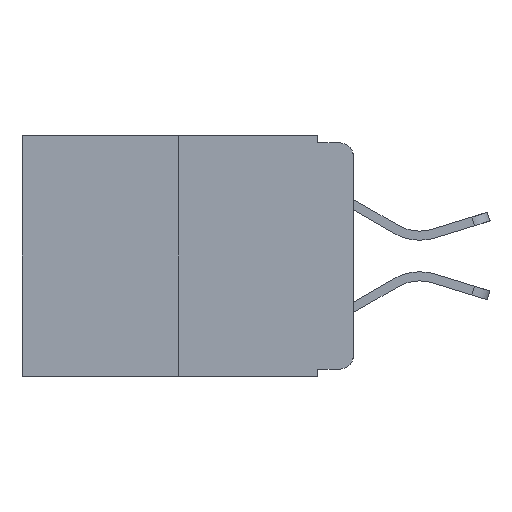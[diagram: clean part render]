
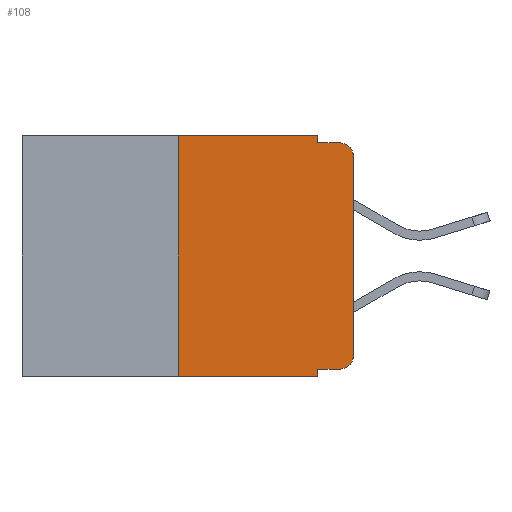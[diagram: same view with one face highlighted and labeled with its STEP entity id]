
A CAD part, left-side view. The second image highlights one B-rep face of the part: STEP entity #108.
In plain terms, the highlighted planar face has unit normal (-1, 0, 0).
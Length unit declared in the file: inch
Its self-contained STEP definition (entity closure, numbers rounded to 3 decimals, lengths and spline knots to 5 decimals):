
#108 = ADVANCED_FACE ( 'NONE', ( #1808 ), #5560, .F. ) ;
#212 = CARTESIAN_POINT ( 'NONE',  ( 0., 0.051, 0. ) ) ;
#527 = CARTESIAN_POINT ( 'NONE',  ( 0., 0.25, 0. ) ) ;
#774 = ORIENTED_EDGE ( 'NONE', *, *, #1072, .F. ) ;
#1025 = EDGE_CURVE ( 'NONE', #7843, #1994, #5682, .T. ) ;
#1051 = EDGE_CURVE ( 'NONE', #1994, #3789, #1605, .T. ) ;
#1071 = EDGE_CURVE ( 'NONE', #3682, #3789, #9269, .T. ) ;
#1072 = EDGE_CURVE ( 'NONE', #5511, #3682, #11808, .T. ) ;
#1080 = ORIENTED_EDGE ( 'NONE', *, *, #1051, .T. ) ;
#1097 = EDGE_CURVE ( 'NONE', #8793, #7537, #13706, .T. ) ;
#1101 = EDGE_CURVE ( 'NONE', #8618, #2497, #8627, .T. ) ;
#1103 = EDGE_CURVE ( 'NONE', #8618, #12869, #2933, .T. ) ;
#1151 = DIRECTION ( 'NONE',  ( 0., 0., -1. ) ) ;
#1175 = EDGE_CURVE ( 'NONE', #12869, #7843, #12238, .T. ) ;
#1605 = CIRCLE ( 'NONE', #10972, 0.02 ) ;
#1808 = FACE_OUTER_BOUND ( 'NONE', #8361, .T. ) ;
#1962 = ORIENTED_EDGE ( 'NONE', *, *, #1071, .F. ) ;
#1994 = VERTEX_POINT ( 'NONE', #10016 ) ;
#2268 = ORIENTED_EDGE ( 'NONE', *, *, #1175, .T. ) ;
#2497 = VERTEX_POINT ( 'NONE', #3131 ) ;
#2572 = VECTOR ( 'NONE', #11953, 39.37008 ) ;
#2722 = ORIENTED_EDGE ( 'NONE', *, *, #3113, .T. ) ;
#2933 = LINE ( 'NONE', #11969, #2572 ) ;
#3113 = EDGE_CURVE ( 'NONE', #8793, #2497, #12500, .T. ) ;
#3131 = CARTESIAN_POINT ( 'NONE',  ( 0., 0.051, -0.343 ) ) ;
#3321 = VECTOR ( 'NONE', #13154, 39.37008 ) ;
#3682 = VERTEX_POINT ( 'NONE', #7727 ) ;
#3704 = CARTESIAN_POINT ( 'NONE',  ( 0., 0.02, -0.03 ) ) ;
#3789 = VERTEX_POINT ( 'NONE', #13698 ) ;
#4072 = DIRECTION ( 'NONE',  ( 0., 0., -1. ) ) ;
#4140 = CARTESIAN_POINT ( 'NONE',  ( 0., 0.051, -0.01 ) ) ;
#4148 = CARTESIAN_POINT ( 'NONE',  ( 0., 0.473, 0. ) ) ;
#4442 = DIRECTION ( 'NONE',  ( -1., 0., 0. ) ) ;
#5148 = CARTESIAN_POINT ( 'NONE',  ( 0., 0.25, -0.343 ) ) ;
#5511 = VERTEX_POINT ( 'NONE', #6146 ) ;
#5560 = PLANE ( 'NONE',  #13375 ) ;
#5682 = LINE ( 'NONE', #12617, #10809 ) ;
#6047 = ORIENTED_EDGE ( 'NONE', *, *, #1025, .T. ) ;
#6146 = CARTESIAN_POINT ( 'NONE',  ( 0., 0.051, 0. ) ) ;
#6204 = DIRECTION ( 'NONE',  ( 0., 0., -1. ) ) ;
#6439 = DIRECTION ( 'NONE',  ( 1., 0., 0. ) ) ;
#6487 = VECTOR ( 'NONE', #9196, 39.37008 ) ;
#6551 = CARTESIAN_POINT ( 'NONE',  ( 0., 0.473, -0.343 ) ) ;
#6746 = CARTESIAN_POINT ( 'NONE',  ( 0., 0., -0.313 ) ) ;
#7527 = EDGE_CURVE ( 'NONE', #7537, #5511, #11515, .T. ) ;
#7537 = VERTEX_POINT ( 'NONE', #527 ) ;
#7670 = CARTESIAN_POINT ( 'NONE',  ( 0., 0.473, 0. ) ) ;
#7727 = CARTESIAN_POINT ( 'NONE',  ( 0., 0.051, -0.01 ) ) ;
#7843 = VERTEX_POINT ( 'NONE', #6746 ) ;
#7930 = CARTESIAN_POINT ( 'NONE',  ( 0., 0.02, -0.333 ) ) ;
#8298 = VECTOR ( 'NONE', #12096, 39.37008 ) ;
#8361 = EDGE_LOOP ( 'NONE', ( #6047, #1080, #1962, #774, #10154, #10473, #2722, #12263, #12125, #2268 ) ) ;
#8618 = VERTEX_POINT ( 'NONE', #9114 ) ;
#8627 = LINE ( 'NONE', #12076, #8298 ) ;
#8793 = VERTEX_POINT ( 'NONE', #5148 ) ;
#9114 = CARTESIAN_POINT ( 'NONE',  ( 0., 0.051, -0.333 ) ) ;
#9196 = DIRECTION ( 'NONE',  ( 0., -1., 0. ) ) ;
#9269 = LINE ( 'NONE', #4140, #6487 ) ;
#9423 = AXIS2_PLACEMENT_3D ( 'NONE', #10462, #10451, #6204 ) ;
#9574 = VECTOR ( 'NONE', #4072, 39.37008 ) ;
#9991 = VECTOR ( 'NONE', #13425, 39.37008 ) ;
#10016 = CARTESIAN_POINT ( 'NONE',  ( 0., 0., -0.03 ) ) ;
#10154 = ORIENTED_EDGE ( 'NONE', *, *, #7527, .F. ) ;
#10451 = DIRECTION ( 'NONE',  ( -1., 0., 0. ) ) ;
#10462 = CARTESIAN_POINT ( 'NONE',  ( 0., 0.02, -0.313 ) ) ;
#10473 = ORIENTED_EDGE ( 'NONE', *, *, #1097, .F. ) ;
#10809 = VECTOR ( 'NONE', #12566, 39.37008 ) ;
#10972 = AXIS2_PLACEMENT_3D ( 'NONE', #3704, #4442, #12277 ) ;
#11515 = LINE ( 'NONE', #4148, #3321 ) ;
#11808 = LINE ( 'NONE', #212, #9574 ) ;
#11953 = DIRECTION ( 'NONE',  ( 0., -1., 0. ) ) ;
#11969 = CARTESIAN_POINT ( 'NONE',  ( 0., 0.051, -0.333 ) ) ;
#12076 = CARTESIAN_POINT ( 'NONE',  ( 0., 0.051, 0. ) ) ;
#12096 = DIRECTION ( 'NONE',  ( 0., 0., -1. ) ) ;
#12109 = CARTESIAN_POINT ( 'NONE',  ( 0., 0.25, 0. ) ) ;
#12125 = ORIENTED_EDGE ( 'NONE', *, *, #1103, .T. ) ;
#12191 = DIRECTION ( 'NONE',  ( 0., 0., 1. ) ) ;
#12238 = CIRCLE ( 'NONE', #9423, 0.02 ) ;
#12263 = ORIENTED_EDGE ( 'NONE', *, *, #1101, .F. ) ;
#12277 = DIRECTION ( 'NONE',  ( 0., 0., -1. ) ) ;
#12500 = LINE ( 'NONE', #6551, #9991 ) ;
#12566 = DIRECTION ( 'NONE',  ( 0., 0., 1. ) ) ;
#12617 = CARTESIAN_POINT ( 'NONE',  ( 0., 0., 0. ) ) ;
#12869 = VERTEX_POINT ( 'NONE', #7930 ) ;
#13154 = DIRECTION ( 'NONE',  ( 0., -1., 0. ) ) ;
#13375 = AXIS2_PLACEMENT_3D ( 'NONE', #7670, #6439, #1151 ) ;
#13410 = VECTOR ( 'NONE', #12191, 39.37008 ) ;
#13425 = DIRECTION ( 'NONE',  ( 0., -1., 0. ) ) ;
#13698 = CARTESIAN_POINT ( 'NONE',  ( 0., 0.02, -0.01 ) ) ;
#13706 = LINE ( 'NONE', #12109, #13410 ) ;
